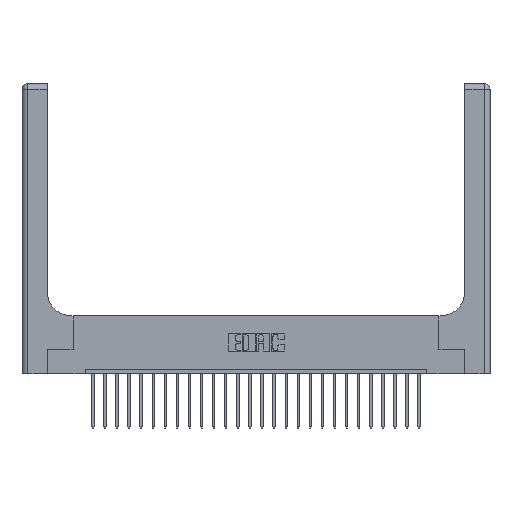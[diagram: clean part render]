
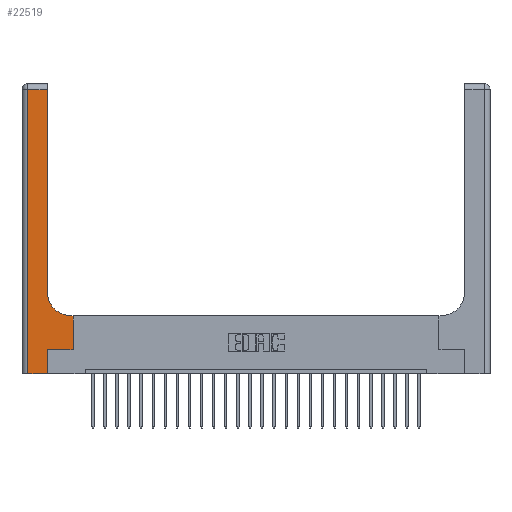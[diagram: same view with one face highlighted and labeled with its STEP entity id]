
A CAD part, top view. The second image highlights one B-rep face of the part: STEP entity #22519.
In plain terms, the highlighted planar face has unit normal (0, 0, 1).
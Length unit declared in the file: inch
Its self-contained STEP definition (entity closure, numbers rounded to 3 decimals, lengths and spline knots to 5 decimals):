
#80 = VERTEX_POINT ( 'NONE', #7503 ) ;
#1606 = VERTEX_POINT ( 'NONE', #20042 ) ;
#2050 = FACE_OUTER_BOUND ( 'NONE', #13032, .T. ) ;
#2353 = DIRECTION ( 'NONE',  ( -1., 0., 0. ) ) ;
#2486 = ORIENTED_EDGE ( 'NONE', *, *, #10576, .T. ) ;
#2600 = LINE ( 'NONE', #19555, #10264 ) ;
#3346 = CARTESIAN_POINT ( 'NONE',  ( 0., 3., 0.37 ) ) ;
#3541 = LINE ( 'NONE', #4569, #18308 ) ;
#3613 = AXIS2_PLACEMENT_3D ( 'NONE', #21600, #19944, #17877 ) ;
#4466 = DIRECTION ( 'NONE',  ( -1., 0., 0. ) ) ;
#4511 = EDGE_CURVE ( 'NONE', #24110, #7171, #15564, .T. ) ;
#4569 = CARTESIAN_POINT ( 'NONE',  ( 0.06, 3., 0.37 ) ) ;
#5227 = CARTESIAN_POINT ( 'NONE',  ( 0.528, 0.25, 0.37 ) ) ;
#5273 = LINE ( 'NONE', #13370, #8223 ) ;
#5633 = VECTOR ( 'NONE', #2353, 39.37008 ) ;
#6712 = DIRECTION ( 'NONE',  ( 0., 1., 0. ) ) ;
#7162 = VECTOR ( 'NONE', #6712, 39.37008 ) ;
#7171 = VERTEX_POINT ( 'NONE', #14344 ) ;
#7293 = CARTESIAN_POINT ( 'NONE',  ( 0.51, 0.6, 0.37 ) ) ;
#7480 = AXIS2_PLACEMENT_3D ( 'NONE', #3346, #24245, #20439 ) ;
#7503 = CARTESIAN_POINT ( 'NONE',  ( 0.06, 0., 0.37 ) ) ;
#7791 = VERTEX_POINT ( 'NONE', #8672 ) ;
#7928 = ORIENTED_EDGE ( 'NONE', *, *, #16500, .T. ) ;
#8223 = VECTOR ( 'NONE', #20745, 39.37008 ) ;
#8672 = CARTESIAN_POINT ( 'NONE',  ( 0.26, 2.94, 0.37 ) ) ;
#10264 = VECTOR ( 'NONE', #4466, 39.37008 ) ;
#10278 = ORIENTED_EDGE ( 'NONE', *, *, #20112, .T. ) ;
#10495 = CIRCLE ( 'NONE', #3613, 0.25 ) ;
#10536 = EDGE_CURVE ( 'NONE', #7791, #21239, #12423, .T. ) ;
#10576 = EDGE_CURVE ( 'NONE', #21239, #80, #3541, .T. ) ;
#10708 = DIRECTION ( 'NONE',  ( 1., 0., 0. ) ) ;
#10807 = CARTESIAN_POINT ( 'NONE',  ( 0.265, 0.25, 0.37 ) ) ;
#10826 = VERTEX_POINT ( 'NONE', #7293 ) ;
#10878 = PLANE ( 'NONE',  #7480 ) ;
#11712 = CARTESIAN_POINT ( 'NONE',  ( 0.265, 0., 0.37 ) ) ;
#12164 = VERTEX_POINT ( 'NONE', #16807 ) ;
#12423 = LINE ( 'NONE', #23055, #5633 ) ;
#13032 = EDGE_LOOP ( 'NONE', ( #21226, #21112, #2486, #16781, #22905, #7928, #17243, #17020, #10278 ) ) ;
#13370 = CARTESIAN_POINT ( 'NONE',  ( 0.528, 0.25, 0.37 ) ) ;
#13804 = VECTOR ( 'NONE', #19044, 39.37008 ) ;
#14344 = CARTESIAN_POINT ( 'NONE',  ( 0.265, 0.25, 0.37 ) ) ;
#15512 = EDGE_CURVE ( 'NONE', #12164, #7791, #21031, .T. ) ;
#15564 = LINE ( 'NONE', #11712, #13804 ) ;
#16433 = LINE ( 'NONE', #18222, #16720 ) ;
#16500 = EDGE_CURVE ( 'NONE', #7171, #23949, #20078, .T. ) ;
#16698 = DIRECTION ( 'NONE',  ( 1., 0., 0. ) ) ;
#16720 = VECTOR ( 'NONE', #10708, 39.37008 ) ;
#16781 = ORIENTED_EDGE ( 'NONE', *, *, #24320, .T. ) ;
#16807 = CARTESIAN_POINT ( 'NONE',  ( 0.26, 0.85, 0.37 ) ) ;
#17020 = ORIENTED_EDGE ( 'NONE', *, *, #18239, .T. ) ;
#17243 = ORIENTED_EDGE ( 'NONE', *, *, #18058, .T. ) ;
#17877 = DIRECTION ( 'NONE',  ( 1., 0., 0. ) ) ;
#18058 = EDGE_CURVE ( 'NONE', #23949, #1606, #5273, .T. ) ;
#18222 = CARTESIAN_POINT ( 'NONE',  ( 0., 0., 0.37 ) ) ;
#18239 = EDGE_CURVE ( 'NONE', #1606, #10826, #2600, .T. ) ;
#18308 = VECTOR ( 'NONE', #21731, 39.37008 ) ;
#19044 = DIRECTION ( 'NONE',  ( 0., 1., 0. ) ) ;
#19200 = VECTOR ( 'NONE', #16698, 39.37008 ) ;
#19301 = CARTESIAN_POINT ( 'NONE',  ( 0.265, 0., 0.37 ) ) ;
#19555 = CARTESIAN_POINT ( 'NONE',  ( 0.26, 0.6, 0.37 ) ) ;
#19944 = DIRECTION ( 'NONE',  ( 0., 0., -1. ) ) ;
#20042 = CARTESIAN_POINT ( 'NONE',  ( 0.528, 0.6, 0.37 ) ) ;
#20078 = LINE ( 'NONE', #10807, #19200 ) ;
#20112 = EDGE_CURVE ( 'NONE', #10826, #12164, #10495, .T. ) ;
#20439 = DIRECTION ( 'NONE',  ( -1., 0., 0. ) ) ;
#20745 = DIRECTION ( 'NONE',  ( 0., 1., 0. ) ) ;
#21031 = LINE ( 'NONE', #22115, #7162 ) ;
#21112 = ORIENTED_EDGE ( 'NONE', *, *, #10536, .T. ) ;
#21226 = ORIENTED_EDGE ( 'NONE', *, *, #15512, .T. ) ;
#21239 = VERTEX_POINT ( 'NONE', #21623 ) ;
#21600 = CARTESIAN_POINT ( 'NONE',  ( 0.51, 0.85, 0.37 ) ) ;
#21623 = CARTESIAN_POINT ( 'NONE',  ( 0.06, 2.94, 0.37 ) ) ;
#21731 = DIRECTION ( 'NONE',  ( 0., -1., 0. ) ) ;
#22115 = CARTESIAN_POINT ( 'NONE',  ( 0.26, 3., 0.37 ) ) ;
#22519 = ADVANCED_FACE ( 'NONE', ( #2050 ), #10878, .F. ) ;
#22905 = ORIENTED_EDGE ( 'NONE', *, *, #4511, .T. ) ;
#23055 = CARTESIAN_POINT ( 'NONE',  ( 0., 2.94, 0.37 ) ) ;
#23949 = VERTEX_POINT ( 'NONE', #5227 ) ;
#24110 = VERTEX_POINT ( 'NONE', #19301 ) ;
#24245 = DIRECTION ( 'NONE',  ( 0., 0., -1. ) ) ;
#24320 = EDGE_CURVE ( 'NONE', #80, #24110, #16433, .T. ) ;
